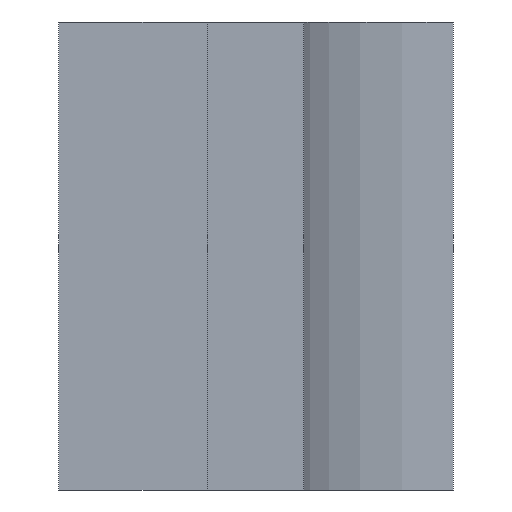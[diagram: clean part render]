
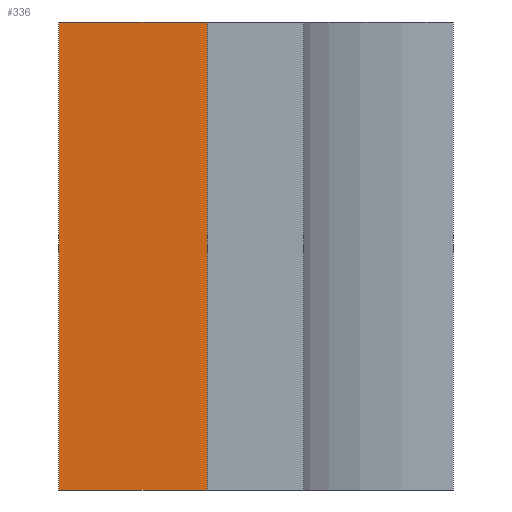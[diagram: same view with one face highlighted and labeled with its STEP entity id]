
A CAD part, front view. The second image highlights one B-rep face of the part: STEP entity #336.
In plain terms, the highlighted planar face has unit normal (0, -1, 0).
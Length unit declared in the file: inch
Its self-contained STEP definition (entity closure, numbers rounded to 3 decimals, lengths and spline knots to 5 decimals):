
#8 = CARTESIAN_POINT ( 'NONE',  ( -0.2, 1., 0.63 ) ) ;
#13 = DIRECTION ( 'NONE',  ( 1., 0., 0. ) ) ;
#20 = CARTESIAN_POINT ( 'NONE',  ( -0.2, 1., 0. ) ) ;
#21 = DIRECTION ( 'NONE',  ( 1., 0., 0. ) ) ;
#26 = DIRECTION ( 'NONE',  ( 1., 0., 0. ) ) ;
#35 = AXIS2_PLACEMENT_3D ( 'NONE', #86, #42, #26 ) ;
#42 = DIRECTION ( 'NONE',  ( 0., -1., 0. ) ) ;
#56 = PLANE ( 'NONE',  #35 ) ;
#75 = ORIENTED_EDGE ( 'NONE', *, *, #153, .T. ) ;
#86 = CARTESIAN_POINT ( 'NONE',  ( -0.2, 1., 0. ) ) ;
#88 = VECTOR ( 'NONE', #21, 39.37008 ) ;
#139 = LINE ( 'NONE', #20, #308 ) ;
#142 = EDGE_CURVE ( 'NONE', #408, #205, #139, .T. ) ;
#146 = ORIENTED_EDGE ( 'NONE', *, *, #233, .F. ) ;
#151 = VECTOR ( 'NONE', #156, 39.37008 ) ;
#153 = EDGE_CURVE ( 'NONE', #205, #341, #318, .T. ) ;
#156 = DIRECTION ( 'NONE',  ( 0., 0., 1. ) ) ;
#159 = CARTESIAN_POINT ( 'NONE',  ( -0.2, 1., 0. ) ) ;
#163 = CARTESIAN_POINT ( 'NONE',  ( 0., 1., 0. ) ) ;
#192 = CARTESIAN_POINT ( 'NONE',  ( -0.2, 1., 0. ) ) ;
#205 = VERTEX_POINT ( 'NONE', #163 ) ;
#208 = CARTESIAN_POINT ( 'NONE',  ( 0., 1., 0.63 ) ) ;
#226 = ORIENTED_EDGE ( 'NONE', *, *, #383, .F. ) ;
#233 = EDGE_CURVE ( 'NONE', #338, #341, #399, .T. ) ;
#249 = CARTESIAN_POINT ( 'NONE',  ( -0.2, 1., 0.63 ) ) ;
#269 = CARTESIAN_POINT ( 'NONE',  ( 0., 1., 0. ) ) ;
#293 = EDGE_LOOP ( 'NONE', ( #75, #146, #226, #310 ) ) ;
#308 = VECTOR ( 'NONE', #13, 39.37008 ) ;
#310 = ORIENTED_EDGE ( 'NONE', *, *, #142, .T. ) ;
#311 = DIRECTION ( 'NONE',  ( 0., 0., 1. ) ) ;
#318 = LINE ( 'NONE', #269, #151 ) ;
#336 = ADVANCED_FACE ( 'NONE', ( #358 ), #56, .T. ) ;
#338 = VERTEX_POINT ( 'NONE', #8 ) ;
#341 = VERTEX_POINT ( 'NONE', #208 ) ;
#346 = VECTOR ( 'NONE', #311, 39.37008 ) ;
#350 = LINE ( 'NONE', #159, #346 ) ;
#358 = FACE_OUTER_BOUND ( 'NONE', #293, .T. ) ;
#383 = EDGE_CURVE ( 'NONE', #408, #338, #350, .T. ) ;
#399 = LINE ( 'NONE', #249, #88 ) ;
#408 = VERTEX_POINT ( 'NONE', #192 ) ;
